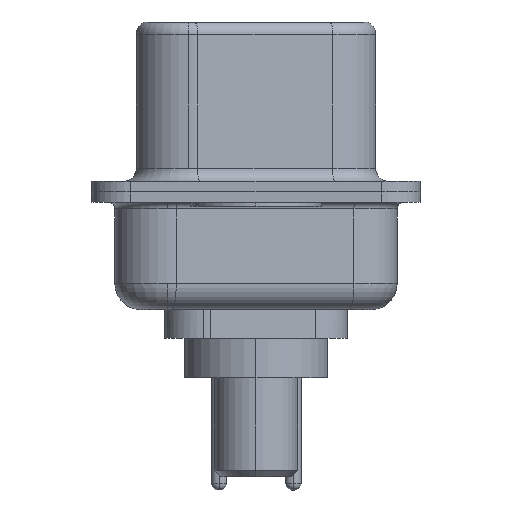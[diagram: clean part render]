
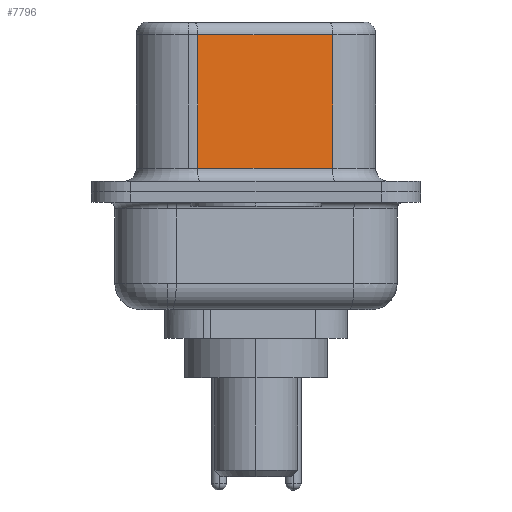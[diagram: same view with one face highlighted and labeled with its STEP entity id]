
A CAD part, left-side view. The second image highlights one B-rep face of the part: STEP entity #7796.
In plain terms, the highlighted planar face has unit normal (-0.985, -0.174, 0).
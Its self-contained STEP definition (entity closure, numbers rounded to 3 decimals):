
#438 = VECTOR ( 'NONE', #7950, 1000. ) ;
#452 = CARTESIAN_POINT ( 'NONE',  ( 3.675, 2.233, 6.02 ) ) ;
#1043 = LINE ( 'NONE', #9138, #11425 ) ;
#1430 = DIRECTION ( 'NONE',  ( 0., 0., -1. ) ) ;
#2366 = VERTEX_POINT ( 'NONE', #12761 ) ;
#2765 = AXIS2_PLACEMENT_3D ( 'NONE', #12414, #4032, #4432 ) ;
#3338 = CARTESIAN_POINT ( 'NONE',  ( 4.585, -2.927, 0.9 ) ) ;
#4032 = DIRECTION ( 'NONE',  ( 0.985, 0.174, 0. ) ) ;
#4432 = DIRECTION ( 'NONE',  ( -0.174, 0.985, 0. ) ) ;
#4698 = DIRECTION ( 'NONE',  ( 0.174, -0.985, 0. ) ) ;
#5878 = CARTESIAN_POINT ( 'NONE',  ( 3.675, 2.233, 0.9 ) ) ;
#6769 = VECTOR ( 'NONE', #4698, 1000. ) ;
#7079 = ORIENTED_EDGE ( 'NONE', *, *, #10662, .T. ) ;
#7796 = ADVANCED_FACE ( 'NONE', ( #11310 ), #8571, .F. ) ;
#7950 = DIRECTION ( 'NONE',  ( -0.174, 0.985, 0. ) ) ;
#8571 = PLANE ( 'NONE',  #2765 ) ;
#9138 = CARTESIAN_POINT ( 'NONE',  ( 3.675, 2.233, 6.52 ) ) ;
#9142 = VERTEX_POINT ( 'NONE', #9458 ) ;
#9458 = CARTESIAN_POINT ( 'NONE',  ( 4.585, -2.927, 6.02 ) ) ;
#9492 = EDGE_CURVE ( 'NONE', #9142, #16188, #10854, .T. ) ;
#9991 = LINE ( 'NONE', #3338, #6769 ) ;
#10473 = DIRECTION ( 'NONE',  ( 0., 0., -1. ) ) ;
#10489 = EDGE_CURVE ( 'NONE', #13614, #2366, #9991, .T. ) ;
#10662 = EDGE_CURVE ( 'NONE', #16188, #13614, #1043, .T. ) ;
#10854 = LINE ( 'NONE', #14734, #438 ) ;
#10994 = ORIENTED_EDGE ( 'NONE', *, *, #10489, .T. ) ;
#11172 = VECTOR ( 'NONE', #1430, 1000. ) ;
#11310 = FACE_OUTER_BOUND ( 'NONE', #15384, .T. ) ;
#11425 = VECTOR ( 'NONE', #10473, 1000. ) ;
#11814 = CARTESIAN_POINT ( 'NONE',  ( 4.585, -2.927, 6.52 ) ) ;
#12287 = EDGE_CURVE ( 'NONE', #9142, #2366, #14798, .T. ) ;
#12414 = CARTESIAN_POINT ( 'NONE',  ( 4.585, -2.927, 6.52 ) ) ;
#12761 = CARTESIAN_POINT ( 'NONE',  ( 4.585, -2.927, 0.9 ) ) ;
#13614 = VERTEX_POINT ( 'NONE', #5878 ) ;
#13770 = ORIENTED_EDGE ( 'NONE', *, *, #9492, .T. ) ;
#14463 = ORIENTED_EDGE ( 'NONE', *, *, #12287, .F. ) ;
#14734 = CARTESIAN_POINT ( 'NONE',  ( 4.585, -2.927, 6.02 ) ) ;
#14798 = LINE ( 'NONE', #11814, #11172 ) ;
#15384 = EDGE_LOOP ( 'NONE', ( #14463, #13770, #7079, #10994 ) ) ;
#16188 = VERTEX_POINT ( 'NONE', #452 ) ;
